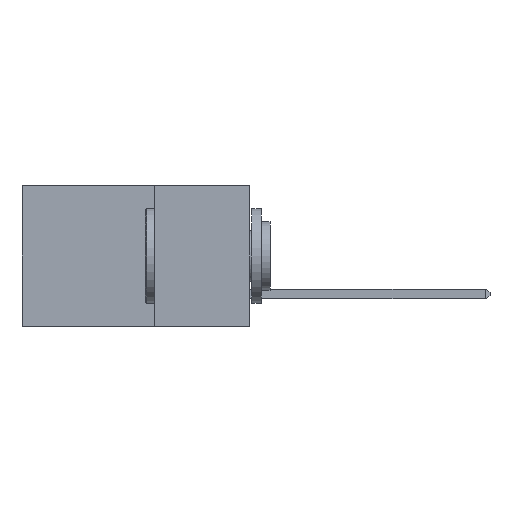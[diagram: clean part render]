
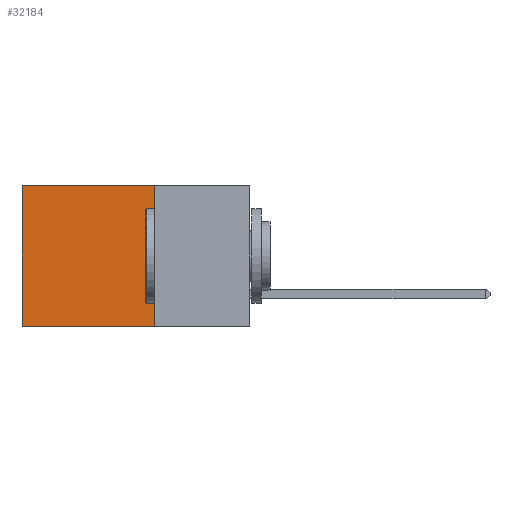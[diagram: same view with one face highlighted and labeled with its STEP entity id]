
A CAD part, left-side view. The second image highlights one B-rep face of the part: STEP entity #32184.
In plain terms, the highlighted planar face has unit normal (-1, 0, 0).
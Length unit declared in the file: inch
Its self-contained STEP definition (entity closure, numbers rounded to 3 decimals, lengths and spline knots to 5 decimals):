
#1955 = CARTESIAN_POINT ( 'NONE',  ( 0.2875, 0.25, -0.37 ) ) ;
#3400 = CARTESIAN_POINT ( 'NONE',  ( 0.2875, 0.25, 0. ) ) ;
#6677 = VECTOR ( 'NONE', #13503, 39.37008 ) ;
#8290 = VERTEX_POINT ( 'NONE', #8914 ) ;
#8914 = CARTESIAN_POINT ( 'NONE',  ( 0.2875, 0.25, 0. ) ) ;
#9207 = LINE ( 'NONE', #36799, #6677 ) ;
#10077 = EDGE_LOOP ( 'NONE', ( #25217, #26076, #31887, #25121 ) ) ;
#10109 = VECTOR ( 'NONE', #29310, 39.37008 ) ;
#11539 = VERTEX_POINT ( 'NONE', #1955 ) ;
#12381 = VERTEX_POINT ( 'NONE', #40963 ) ;
#13503 = DIRECTION ( 'NONE',  ( 0., 0., -1. ) ) ;
#20558 = EDGE_CURVE ( 'NONE', #8290, #28769, #37693, .T. ) ;
#21485 = CARTESIAN_POINT ( 'NONE',  ( 0.2875, 0.25, 0. ) ) ;
#25121 = ORIENTED_EDGE ( 'NONE', *, *, #20558, .T. ) ;
#25217 = ORIENTED_EDGE ( 'NONE', *, *, #34635, .T. ) ;
#26076 = ORIENTED_EDGE ( 'NONE', *, *, #40998, .F. ) ;
#26626 = CARTESIAN_POINT ( 'NONE',  ( 0.2875, 0.6, 0. ) ) ;
#27959 = CARTESIAN_POINT ( 'NONE',  ( 0.2875, 0.6, 0. ) ) ;
#28480 = PLANE ( 'NONE',  #36873 ) ;
#28769 = VERTEX_POINT ( 'NONE', #26626 ) ;
#29310 = DIRECTION ( 'NONE',  ( 0., 1., 0. ) ) ;
#30533 = VECTOR ( 'NONE', #31587, 39.37008 ) ;
#30634 = LINE ( 'NONE', #27959, #31144 ) ;
#31144 = VECTOR ( 'NONE', #37800, 39.37008 ) ;
#31587 = DIRECTION ( 'NONE',  ( 0., 1., 0. ) ) ;
#31887 = ORIENTED_EDGE ( 'NONE', *, *, #34271, .F. ) ;
#32184 = ADVANCED_FACE ( 'NONE', ( #35485 ), #28480, .F. ) ;
#34271 = EDGE_CURVE ( 'NONE', #8290, #11539, #9207, .T. ) ;
#34635 = EDGE_CURVE ( 'NONE', #28769, #12381, #30634, .T. ) ;
#35485 = FACE_OUTER_BOUND ( 'NONE', #10077, .T. ) ;
#36799 = CARTESIAN_POINT ( 'NONE',  ( 0.2875, 0.25, 0. ) ) ;
#36873 = AXIS2_PLACEMENT_3D ( 'NONE', #21485, #38035, #41004 ) ;
#37693 = LINE ( 'NONE', #3400, #10109 ) ;
#37800 = DIRECTION ( 'NONE',  ( 0., 0., -1. ) ) ;
#38035 = DIRECTION ( 'NONE',  ( 1., 0., 0. ) ) ;
#40963 = CARTESIAN_POINT ( 'NONE',  ( 0.2875, 0.6, -0.37 ) ) ;
#40998 = EDGE_CURVE ( 'NONE', #11539, #12381, #41253, .T. ) ;
#41004 = DIRECTION ( 'NONE',  ( 0., 0., -1. ) ) ;
#41253 = LINE ( 'NONE', #41669, #30533 ) ;
#41669 = CARTESIAN_POINT ( 'NONE',  ( 0.2875, 0.25, -0.37 ) ) ;
